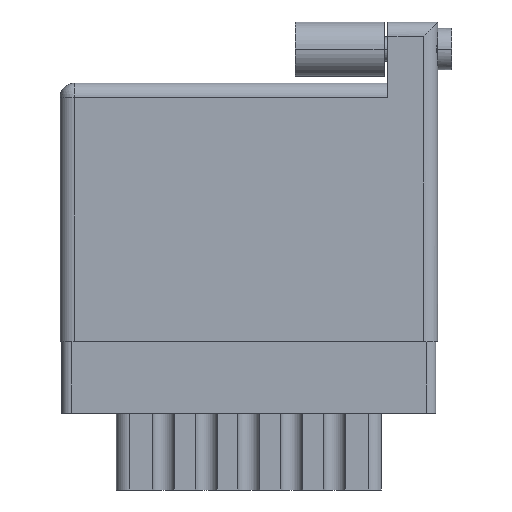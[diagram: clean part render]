
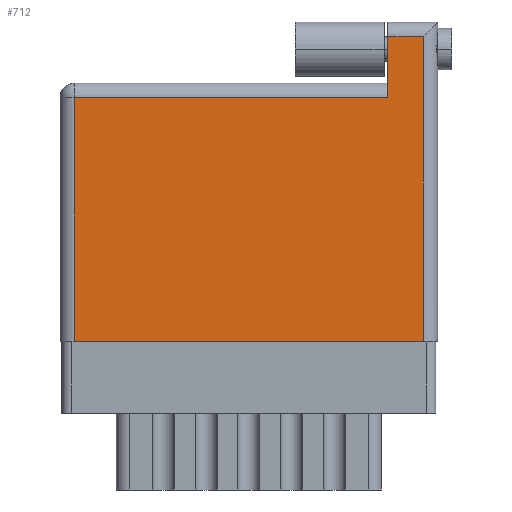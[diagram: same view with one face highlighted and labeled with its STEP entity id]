
A CAD part, front view. The second image highlights one B-rep face of the part: STEP entity #712.
In plain terms, the highlighted face is planar.
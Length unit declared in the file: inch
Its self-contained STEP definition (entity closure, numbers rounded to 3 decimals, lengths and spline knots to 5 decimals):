
#712 = ADVANCED_FACE ( 'NONE', ( #892 ), #20240, .F. ) ;
#892 = FACE_OUTER_BOUND ( 'NONE', #12698, .T. ) ;
#947 = CARTESIAN_POINT ( 'NONE',  ( 1.275, 0., 0. ) ) ;
#2256 = CARTESIAN_POINT ( 'NONE',  ( 1.15, 0.856, 0. ) ) ;
#2304 = EDGE_CURVE ( 'NONE', #14008, #22535, #17501, .T. ) ;
#2716 = DIRECTION ( 'NONE',  ( -1., 0., 0. ) ) ;
#4279 = VECTOR ( 'NONE', #4985, 39.37008 ) ;
#4351 = CARTESIAN_POINT ( 'NONE',  ( 0., 0., 0. ) ) ;
#4417 = CARTESIAN_POINT ( 'NONE',  ( 0., 0.906, 0. ) ) ;
#4477 = CARTESIAN_POINT ( 'NONE',  ( 0.05, 0., 0. ) ) ;
#4985 = DIRECTION ( 'NONE',  ( 0., 1., 0. ) ) ;
#6308 = DIRECTION ( 'NONE',  ( 0., -1., 0. ) ) ;
#6523 = VECTOR ( 'NONE', #11223, 39.37008 ) ;
#7314 = CARTESIAN_POINT ( 'NONE',  ( 0., 1.07, 0. ) ) ;
#7565 = VECTOR ( 'NONE', #7921, 39.37008 ) ;
#7892 = EDGE_CURVE ( 'NONE', #13886, #15460, #9970, .T. ) ;
#7921 = DIRECTION ( 'NONE',  ( 0., -1., 0. ) ) ;
#8316 = VERTEX_POINT ( 'NONE', #12402 ) ;
#8676 = EDGE_CURVE ( 'NONE', #9133, #14008, #19076, .T. ) ;
#9133 = VERTEX_POINT ( 'NONE', #11572 ) ;
#9523 = CARTESIAN_POINT ( 'NONE',  ( 0., 0.856, 0. ) ) ;
#9970 = LINE ( 'NONE', #4351, #14003 ) ;
#10160 = ORIENTED_EDGE ( 'NONE', *, *, #2304, .T. ) ;
#10354 = ORIENTED_EDGE ( 'NONE', *, *, #24675, .T. ) ;
#10836 = EDGE_CURVE ( 'NONE', #15460, #9133, #17161, .T. ) ;
#11223 = DIRECTION ( 'NONE',  ( -1., 0., 0. ) ) ;
#11313 = ORIENTED_EDGE ( 'NONE', *, *, #16447, .T. ) ;
#11572 = CARTESIAN_POINT ( 'NONE',  ( 1.275, 1.07, 0. ) ) ;
#12313 = ORIENTED_EDGE ( 'NONE', *, *, #10836, .T. ) ;
#12402 = CARTESIAN_POINT ( 'NONE',  ( 0.05, 0.856, 0. ) ) ;
#12698 = EDGE_LOOP ( 'NONE', ( #24188, #12313, #22062, #10160, #10354, #11313 ) ) ;
#13184 = DIRECTION ( 'NONE',  ( -1., 0., 0. ) ) ;
#13886 = VERTEX_POINT ( 'NONE', #24614 ) ;
#14003 = VECTOR ( 'NONE', #14153, 39.37008 ) ;
#14008 = VERTEX_POINT ( 'NONE', #25602 ) ;
#14153 = DIRECTION ( 'NONE',  ( 1., 0., 0. ) ) ;
#15393 = CARTESIAN_POINT ( 'NONE',  ( 1.15, 1.12, 0. ) ) ;
#15460 = VERTEX_POINT ( 'NONE', #947 ) ;
#16264 = LINE ( 'NONE', #4477, #20956 ) ;
#16447 = EDGE_CURVE ( 'NONE', #8316, #13886, #16264, .T. ) ;
#17161 = LINE ( 'NONE', #18251, #4279 ) ;
#17501 = LINE ( 'NONE', #15393, #7565 ) ;
#18251 = CARTESIAN_POINT ( 'NONE',  ( 1.275, 1.12, 0. ) ) ;
#19076 = LINE ( 'NONE', #7314, #6523 ) ;
#20240 = PLANE ( 'NONE',  #21005 ) ;
#20241 = VECTOR ( 'NONE', #13184, 39.37008 ) ;
#20956 = VECTOR ( 'NONE', #6308, 39.37008 ) ;
#21005 = AXIS2_PLACEMENT_3D ( 'NONE', #4417, #24302, #2716 ) ;
#22062 = ORIENTED_EDGE ( 'NONE', *, *, #8676, .T. ) ;
#22535 = VERTEX_POINT ( 'NONE', #2256 ) ;
#24188 = ORIENTED_EDGE ( 'NONE', *, *, #7892, .T. ) ;
#24302 = DIRECTION ( 'NONE',  ( 0., 0., -1. ) ) ;
#24614 = CARTESIAN_POINT ( 'NONE',  ( 0.05, 0., 0. ) ) ;
#24675 = EDGE_CURVE ( 'NONE', #22535, #8316, #25495, .T. ) ;
#25495 = LINE ( 'NONE', #9523, #20241 ) ;
#25602 = CARTESIAN_POINT ( 'NONE',  ( 1.15, 1.07, 0. ) ) ;
